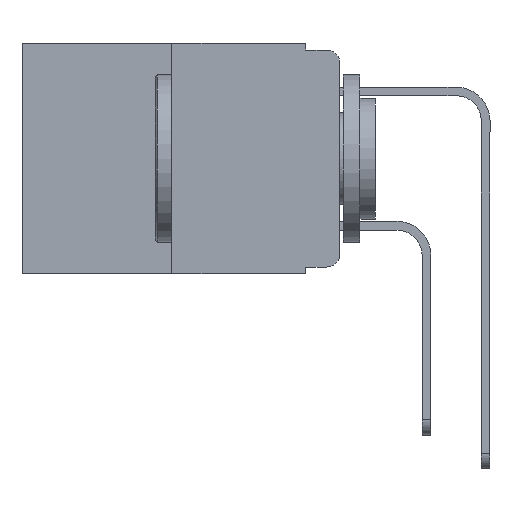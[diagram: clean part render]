
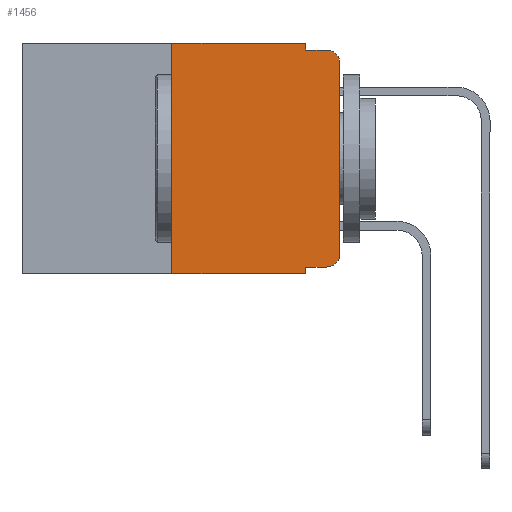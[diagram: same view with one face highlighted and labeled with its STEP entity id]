
A CAD part, left-side view. The second image highlights one B-rep face of the part: STEP entity #1456.
In plain terms, the highlighted planar face has unit normal (-1, 0, 0).
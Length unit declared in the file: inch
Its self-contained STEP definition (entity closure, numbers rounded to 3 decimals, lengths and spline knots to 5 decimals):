
#5 = VECTOR ( 'NONE', #11736, 39.37008 ) ;
#132 = DIRECTION ( 'NONE',  ( -1., 0., 0. ) ) ;
#192 = CARTESIAN_POINT ( 'NONE',  ( 0., 0.051, 0. ) ) ;
#316 = CARTESIAN_POINT ( 'NONE',  ( 0., 0.473, 0. ) ) ;
#320 = VERTEX_POINT ( 'NONE', #6250 ) ;
#491 = EDGE_CURVE ( 'NONE', #10651, #320, #6728, .T. ) ;
#1273 = EDGE_CURVE ( 'NONE', #10651, #14233, #7816, .T. ) ;
#1456 = ADVANCED_FACE ( 'NONE', ( #11378 ), #11092, .F. ) ;
#1490 = VECTOR ( 'NONE', #14587, 39.37008 ) ;
#1584 = VECTOR ( 'NONE', #12394, 39.37008 ) ;
#1724 = VERTEX_POINT ( 'NONE', #192 ) ;
#1852 = ORIENTED_EDGE ( 'NONE', *, *, #5561, .F. ) ;
#2404 = VECTOR ( 'NONE', #5049, 39.37008 ) ;
#2783 = ORIENTED_EDGE ( 'NONE', *, *, #14674, .T. ) ;
#3053 = VERTEX_POINT ( 'NONE', #5097 ) ;
#3573 = EDGE_CURVE ( 'NONE', #5395, #5747, #12383, .T. ) ;
#3712 = CARTESIAN_POINT ( 'NONE',  ( 0., 0.25, -0.343 ) ) ;
#3960 = VECTOR ( 'NONE', #5785, 39.37008 ) ;
#4058 = VECTOR ( 'NONE', #14364, 39.37008 ) ;
#4060 = AXIS2_PLACEMENT_3D ( 'NONE', #316, #8736, #8734 ) ;
#4268 = ORIENTED_EDGE ( 'NONE', *, *, #1273, .F. ) ;
#4324 = CARTESIAN_POINT ( 'NONE',  ( 0., 0.051, 0. ) ) ;
#4356 = EDGE_CURVE ( 'NONE', #1724, #11887, #5493, .T. ) ;
#4530 = LINE ( 'NONE', #8905, #1490 ) ;
#4714 = CIRCLE ( 'NONE', #8866, 0.02 ) ;
#4781 = DIRECTION ( 'NONE',  ( 0., -1., 0. ) ) ;
#5049 = DIRECTION ( 'NONE',  ( 0., 0., -1. ) ) ;
#5097 = CARTESIAN_POINT ( 'NONE',  ( 0., 0., -0.313 ) ) ;
#5138 = EDGE_CURVE ( 'NONE', #11887, #12341, #4530, .T. ) ;
#5395 = VERTEX_POINT ( 'NONE', #3712 ) ;
#5493 = LINE ( 'NONE', #12013, #2404 ) ;
#5561 = EDGE_CURVE ( 'NONE', #5747, #1724, #11095, .T. ) ;
#5696 = ORIENTED_EDGE ( 'NONE', *, *, #3573, .F. ) ;
#5747 = VERTEX_POINT ( 'NONE', #6752 ) ;
#5785 = DIRECTION ( 'NONE',  ( 0., 0., 1. ) ) ;
#5960 = EDGE_CURVE ( 'NONE', #11675, #12341, #6597, .T. ) ;
#6250 = CARTESIAN_POINT ( 'NONE',  ( 0., 0.02, -0.333 ) ) ;
#6434 = DIRECTION ( 'NONE',  ( -1., 0., 0. ) ) ;
#6597 = CIRCLE ( 'NONE', #14565, 0.02 ) ;
#6610 = ORIENTED_EDGE ( 'NONE', *, *, #5138, .F. ) ;
#6728 = LINE ( 'NONE', #9961, #10186 ) ;
#6752 = CARTESIAN_POINT ( 'NONE',  ( 0., 0.25, 0. ) ) ;
#7167 = CARTESIAN_POINT ( 'NONE',  ( 0., 0.02, -0.03 ) ) ;
#7555 = EDGE_CURVE ( 'NONE', #3053, #11675, #12492, .T. ) ;
#7565 = CARTESIAN_POINT ( 'NONE',  ( 0., 0.473, -0.343 ) ) ;
#7736 = ORIENTED_EDGE ( 'NONE', *, *, #7555, .T. ) ;
#7816 = LINE ( 'NONE', #4324, #1584 ) ;
#7945 = LINE ( 'NONE', #7565, #4058 ) ;
#7984 = ORIENTED_EDGE ( 'NONE', *, *, #491, .T. ) ;
#8173 = CARTESIAN_POINT ( 'NONE',  ( 0., 0., 0. ) ) ;
#8342 = DIRECTION ( 'NONE',  ( 0., 0., -1. ) ) ;
#8412 = VECTOR ( 'NONE', #13214, 39.37008 ) ;
#8734 = DIRECTION ( 'NONE',  ( 0., 0., -1. ) ) ;
#8736 = DIRECTION ( 'NONE',  ( 1., 0., 0. ) ) ;
#8767 = CARTESIAN_POINT ( 'NONE',  ( 0., 0.051, -0.01 ) ) ;
#8866 = AXIS2_PLACEMENT_3D ( 'NONE', #13294, #6434, #14416 ) ;
#8905 = CARTESIAN_POINT ( 'NONE',  ( 0., 0.051, -0.01 ) ) ;
#9870 = CARTESIAN_POINT ( 'NONE',  ( 0., 0.473, 0. ) ) ;
#9961 = CARTESIAN_POINT ( 'NONE',  ( 0., 0.051, -0.333 ) ) ;
#10186 = VECTOR ( 'NONE', #4781, 39.37008 ) ;
#10651 = VERTEX_POINT ( 'NONE', #14248 ) ;
#10765 = ORIENTED_EDGE ( 'NONE', *, *, #4356, .F. ) ;
#10783 = ORIENTED_EDGE ( 'NONE', *, *, #5960, .T. ) ;
#11092 = PLANE ( 'NONE',  #4060 ) ;
#11095 = LINE ( 'NONE', #9870, #8412 ) ;
#11365 = EDGE_LOOP ( 'NONE', ( #7736, #10783, #6610, #10765, #1852, #5696, #13195, #4268, #7984, #2783 ) ) ;
#11378 = FACE_OUTER_BOUND ( 'NONE', #11365, .T. ) ;
#11675 = VERTEX_POINT ( 'NONE', #11811 ) ;
#11736 = DIRECTION ( 'NONE',  ( 0., 0., 1. ) ) ;
#11811 = CARTESIAN_POINT ( 'NONE',  ( 0., 0., -0.03 ) ) ;
#11887 = VERTEX_POINT ( 'NONE', #8767 ) ;
#12013 = CARTESIAN_POINT ( 'NONE',  ( 0., 0.051, 0. ) ) ;
#12341 = VERTEX_POINT ( 'NONE', #13452 ) ;
#12383 = LINE ( 'NONE', #13956, #5 ) ;
#12394 = DIRECTION ( 'NONE',  ( 0., 0., -1. ) ) ;
#12492 = LINE ( 'NONE', #8173, #3960 ) ;
#13195 = ORIENTED_EDGE ( 'NONE', *, *, #13367, .T. ) ;
#13214 = DIRECTION ( 'NONE',  ( 0., -1., 0. ) ) ;
#13294 = CARTESIAN_POINT ( 'NONE',  ( 0., 0.02, -0.313 ) ) ;
#13367 = EDGE_CURVE ( 'NONE', #5395, #14233, #7945, .T. ) ;
#13452 = CARTESIAN_POINT ( 'NONE',  ( 0., 0.02, -0.01 ) ) ;
#13585 = CARTESIAN_POINT ( 'NONE',  ( 0., 0.051, -0.343 ) ) ;
#13956 = CARTESIAN_POINT ( 'NONE',  ( 0., 0.25, 0. ) ) ;
#14233 = VERTEX_POINT ( 'NONE', #13585 ) ;
#14248 = CARTESIAN_POINT ( 'NONE',  ( 0., 0.051, -0.333 ) ) ;
#14364 = DIRECTION ( 'NONE',  ( 0., -1., 0. ) ) ;
#14416 = DIRECTION ( 'NONE',  ( 0., 0., -1. ) ) ;
#14565 = AXIS2_PLACEMENT_3D ( 'NONE', #7167, #132, #8342 ) ;
#14587 = DIRECTION ( 'NONE',  ( 0., -1., 0. ) ) ;
#14674 = EDGE_CURVE ( 'NONE', #320, #3053, #4714, .T. ) ;
